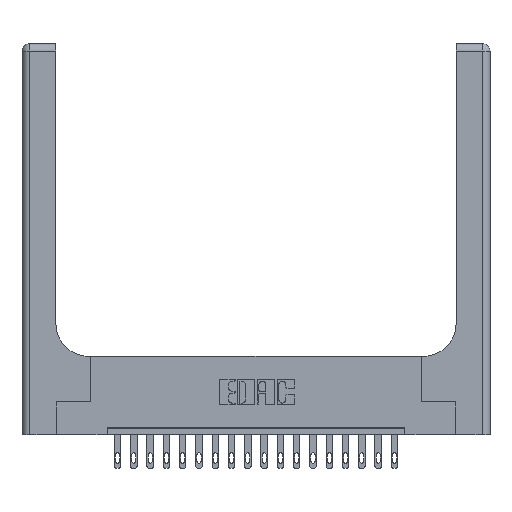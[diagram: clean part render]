
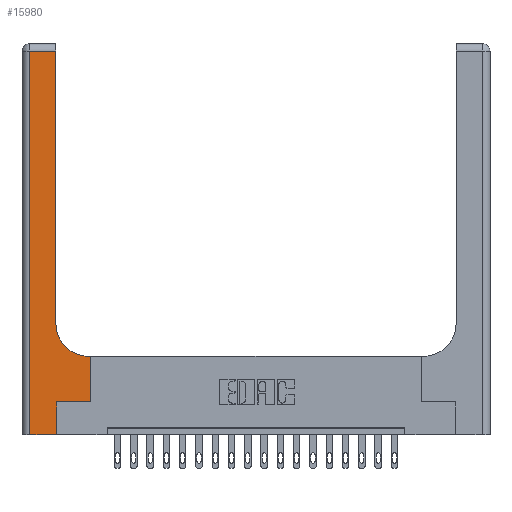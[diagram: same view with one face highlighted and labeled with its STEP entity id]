
A CAD part, top view. The second image highlights one B-rep face of the part: STEP entity #15980.
In plain terms, the highlighted planar face has unit normal (0, 0, 1).
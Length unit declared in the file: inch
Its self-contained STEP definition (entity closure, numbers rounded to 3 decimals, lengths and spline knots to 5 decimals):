
#48 = ORIENTED_EDGE ( 'NONE', *, *, #19471, .T. ) ;
#197 = DIRECTION ( 'NONE',  ( 1., 0., 0. ) ) ;
#388 = CARTESIAN_POINT ( 'NONE',  ( 0.26, 0.6, 0.37 ) ) ;
#697 = ORIENTED_EDGE ( 'NONE', *, *, #14981, .T. ) ;
#877 = CARTESIAN_POINT ( 'NONE',  ( 0.06, 0., 0.37 ) ) ;
#1224 = VECTOR ( 'NONE', #18124, 39.37008 ) ;
#1440 = CARTESIAN_POINT ( 'NONE',  ( 0.26, 0.85, 0.37 ) ) ;
#2367 = PLANE ( 'NONE',  #7725 ) ;
#2550 = AXIS2_PLACEMENT_3D ( 'NONE', #15591, #12558, #17101 ) ;
#2596 = DIRECTION ( 'NONE',  ( 1., 0., 0. ) ) ;
#2693 = LINE ( 'NONE', #5707, #14428 ) ;
#2821 = VERTEX_POINT ( 'NONE', #16949 ) ;
#3436 = VECTOR ( 'NONE', #16449, 39.37008 ) ;
#3880 = FACE_OUTER_BOUND ( 'NONE', #13770, .T. ) ;
#3954 = EDGE_CURVE ( 'NONE', #12718, #18194, #6546, .T. ) ;
#4306 = LINE ( 'NONE', #10273, #5708 ) ;
#5143 = ORIENTED_EDGE ( 'NONE', *, *, #17458, .T. ) ;
#5707 = CARTESIAN_POINT ( 'NONE',  ( 0.26, 3., 0.37 ) ) ;
#5708 = VECTOR ( 'NONE', #2596, 39.37008 ) ;
#6219 = ORIENTED_EDGE ( 'NONE', *, *, #13522, .T. ) ;
#6466 = VECTOR ( 'NONE', #6882, 39.37008 ) ;
#6546 = LINE ( 'NONE', #18578, #19196 ) ;
#6882 = DIRECTION ( 'NONE',  ( -1., 0., 0. ) ) ;
#7663 = VECTOR ( 'NONE', #18297, 39.37008 ) ;
#7725 = AXIS2_PLACEMENT_3D ( 'NONE', #12887, #8518, #8322 ) ;
#7827 = EDGE_CURVE ( 'NONE', #19785, #12718, #14843, .T. ) ;
#7983 = VERTEX_POINT ( 'NONE', #11995 ) ;
#8038 = CARTESIAN_POINT ( 'NONE',  ( 0.26, 2.94, 0.37 ) ) ;
#8229 = VERTEX_POINT ( 'NONE', #8038 ) ;
#8322 = DIRECTION ( 'NONE',  ( -1., 0., 0. ) ) ;
#8349 = CIRCLE ( 'NONE', #2550, 0.25 ) ;
#8358 = VERTEX_POINT ( 'NONE', #877 ) ;
#8518 = DIRECTION ( 'NONE',  ( 0., 0., -1. ) ) ;
#9259 = ORIENTED_EDGE ( 'NONE', *, *, #13131, .T. ) ;
#9978 = VERTEX_POINT ( 'NONE', #1440 ) ;
#10185 = CARTESIAN_POINT ( 'NONE',  ( 0.265, 0., 0.37 ) ) ;
#10273 = CARTESIAN_POINT ( 'NONE',  ( 0., 0., 0.37 ) ) ;
#10718 = CARTESIAN_POINT ( 'NONE',  ( 0.528, 0.25, 0.37 ) ) ;
#10770 = EDGE_CURVE ( 'NONE', #9978, #8229, #2693, .T. ) ;
#11443 = CARTESIAN_POINT ( 'NONE',  ( 0., 2.94, 0.37 ) ) ;
#11567 = ORIENTED_EDGE ( 'NONE', *, *, #14067, .T. ) ;
#11995 = CARTESIAN_POINT ( 'NONE',  ( 0.528, 0.6, 0.37 ) ) ;
#12300 = VECTOR ( 'NONE', #18662, 39.37008 ) ;
#12321 = CARTESIAN_POINT ( 'NONE',  ( 0.528, 0.25, 0.37 ) ) ;
#12558 = DIRECTION ( 'NONE',  ( 0., 0., -1. ) ) ;
#12718 = VERTEX_POINT ( 'NONE', #14177 ) ;
#12721 = VERTEX_POINT ( 'NONE', #14277 ) ;
#12837 = ORIENTED_EDGE ( 'NONE', *, *, #3954, .T. ) ;
#12887 = CARTESIAN_POINT ( 'NONE',  ( 0., 3., 0.37 ) ) ;
#13131 = EDGE_CURVE ( 'NONE', #8358, #19785, #4306, .T. ) ;
#13287 = LINE ( 'NONE', #15203, #1224 ) ;
#13406 = DIRECTION ( 'NONE',  ( 0., 1., 0. ) ) ;
#13522 = EDGE_CURVE ( 'NONE', #2821, #8358, #13287, .T. ) ;
#13762 = LINE ( 'NONE', #10718, #7663 ) ;
#13770 = EDGE_LOOP ( 'NONE', ( #14689, #5143, #6219, #9259, #19729, #12837, #11567, #48, #697 ) ) ;
#14067 = EDGE_CURVE ( 'NONE', #18194, #7983, #13762, .T. ) ;
#14177 = CARTESIAN_POINT ( 'NONE',  ( 0.265, 0.25, 0.37 ) ) ;
#14277 = CARTESIAN_POINT ( 'NONE',  ( 0.51, 0.6, 0.37 ) ) ;
#14428 = VECTOR ( 'NONE', #13406, 39.37008 ) ;
#14689 = ORIENTED_EDGE ( 'NONE', *, *, #10770, .T. ) ;
#14843 = LINE ( 'NONE', #10185, #3436 ) ;
#14981 = EDGE_CURVE ( 'NONE', #12721, #9978, #8349, .T. ) ;
#15203 = CARTESIAN_POINT ( 'NONE',  ( 0.06, 3., 0.37 ) ) ;
#15496 = CARTESIAN_POINT ( 'NONE',  ( 0.265, 0., 0.37 ) ) ;
#15591 = CARTESIAN_POINT ( 'NONE',  ( 0.51, 0.85, 0.37 ) ) ;
#15980 = ADVANCED_FACE ( 'NONE', ( #3880 ), #2367, .F. ) ;
#16449 = DIRECTION ( 'NONE',  ( 0., 1., 0. ) ) ;
#16949 = CARTESIAN_POINT ( 'NONE',  ( 0.06, 2.94, 0.37 ) ) ;
#17101 = DIRECTION ( 'NONE',  ( 1., 0., 0. ) ) ;
#17354 = LINE ( 'NONE', #388, #12300 ) ;
#17458 = EDGE_CURVE ( 'NONE', #8229, #2821, #19207, .T. ) ;
#18124 = DIRECTION ( 'NONE',  ( 0., -1., 0. ) ) ;
#18194 = VERTEX_POINT ( 'NONE', #12321 ) ;
#18297 = DIRECTION ( 'NONE',  ( 0., 1., 0. ) ) ;
#18578 = CARTESIAN_POINT ( 'NONE',  ( 0.265, 0.25, 0.37 ) ) ;
#18662 = DIRECTION ( 'NONE',  ( -1., 0., 0. ) ) ;
#19196 = VECTOR ( 'NONE', #197, 39.37008 ) ;
#19207 = LINE ( 'NONE', #11443, #6466 ) ;
#19471 = EDGE_CURVE ( 'NONE', #7983, #12721, #17354, .T. ) ;
#19729 = ORIENTED_EDGE ( 'NONE', *, *, #7827, .T. ) ;
#19785 = VERTEX_POINT ( 'NONE', #15496 ) ;
